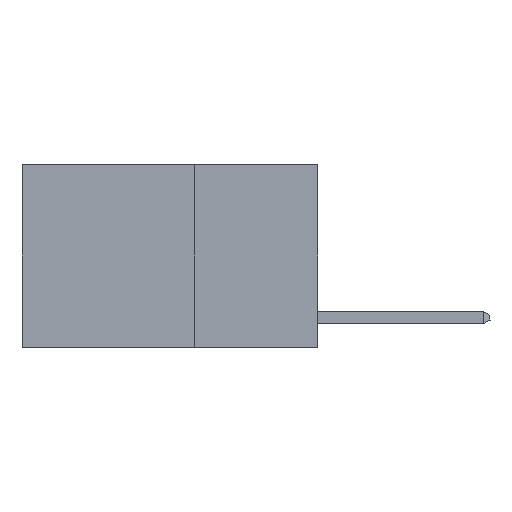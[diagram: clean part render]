
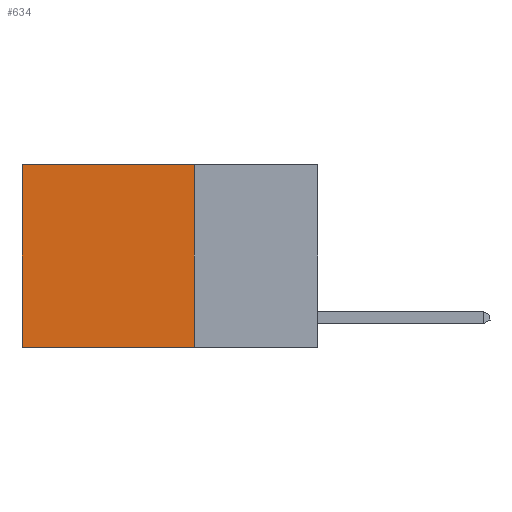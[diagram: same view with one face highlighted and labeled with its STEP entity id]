
A CAD part, left-side view. The second image highlights one B-rep face of the part: STEP entity #634.
In plain terms, the highlighted planar face has unit normal (-1, 0, 0).
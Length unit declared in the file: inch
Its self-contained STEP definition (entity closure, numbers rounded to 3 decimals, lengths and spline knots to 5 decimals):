
#634 = ADVANCED_FACE ( 'NONE', ( #9609 ), #5693, .F. ) ;
#1008 = ORIENTED_EDGE ( 'NONE', *, *, #11828, .T. ) ;
#1025 = VERTEX_POINT ( 'NONE', #1209 ) ;
#1051 = DIRECTION ( 'NONE',  ( 0., 0., -1. ) ) ;
#1209 = CARTESIAN_POINT ( 'NONE',  ( 0.2625, 0.25, 0. ) ) ;
#3025 = LINE ( 'NONE', #24313, #7670 ) ;
#3166 = ORIENTED_EDGE ( 'NONE', *, *, #4127, .F. ) ;
#3971 = VECTOR ( 'NONE', #21203, 39.37008 ) ;
#4127 = EDGE_CURVE ( 'NONE', #1025, #20558, #14402, .T. ) ;
#4429 = CARTESIAN_POINT ( 'NONE',  ( 0.2625, 0.6, 0. ) ) ;
#5693 = PLANE ( 'NONE',  #18815 ) ;
#6314 = EDGE_LOOP ( 'NONE', ( #21284, #13641, #3166, #1008 ) ) ;
#7668 = DIRECTION ( 'NONE',  ( 1., 0., 0. ) ) ;
#7670 = VECTOR ( 'NONE', #10549, 39.37008 ) ;
#8001 = CARTESIAN_POINT ( 'NONE',  ( 0.2625, 0.25, -0.37 ) ) ;
#8842 = VERTEX_POINT ( 'NONE', #14545 ) ;
#9609 = FACE_OUTER_BOUND ( 'NONE', #6314, .T. ) ;
#10325 = DIRECTION ( 'NONE',  ( 0., 0., -1. ) ) ;
#10549 = DIRECTION ( 'NONE',  ( 0., 1., 0. ) ) ;
#11828 = EDGE_CURVE ( 'NONE', #1025, #13928, #3025, .T. ) ;
#12011 = VECTOR ( 'NONE', #10325, 39.37008 ) ;
#12936 = CARTESIAN_POINT ( 'NONE',  ( 0.2625, 0.25, 0. ) ) ;
#13641 = ORIENTED_EDGE ( 'NONE', *, *, #14943, .F. ) ;
#13928 = VERTEX_POINT ( 'NONE', #24207 ) ;
#14402 = LINE ( 'NONE', #12936, #24872 ) ;
#14545 = CARTESIAN_POINT ( 'NONE',  ( 0.2625, 0.6, -0.37 ) ) ;
#14943 = EDGE_CURVE ( 'NONE', #20558, #8842, #24961, .T. ) ;
#18815 = AXIS2_PLACEMENT_3D ( 'NONE', #19431, #7668, #21413 ) ;
#19215 = CARTESIAN_POINT ( 'NONE',  ( 0.2625, 0.25, -0.37 ) ) ;
#19431 = CARTESIAN_POINT ( 'NONE',  ( 0.2625, 0.25, 0. ) ) ;
#20558 = VERTEX_POINT ( 'NONE', #8001 ) ;
#21203 = DIRECTION ( 'NONE',  ( 0., 1., 0. ) ) ;
#21284 = ORIENTED_EDGE ( 'NONE', *, *, #24215, .T. ) ;
#21413 = DIRECTION ( 'NONE',  ( 0., 0., -1. ) ) ;
#22436 = LINE ( 'NONE', #4429, #12011 ) ;
#24207 = CARTESIAN_POINT ( 'NONE',  ( 0.2625, 0.6, 0. ) ) ;
#24215 = EDGE_CURVE ( 'NONE', #13928, #8842, #22436, .T. ) ;
#24313 = CARTESIAN_POINT ( 'NONE',  ( 0.2625, 0.25, 0. ) ) ;
#24872 = VECTOR ( 'NONE', #1051, 39.37008 ) ;
#24961 = LINE ( 'NONE', #19215, #3971 ) ;
